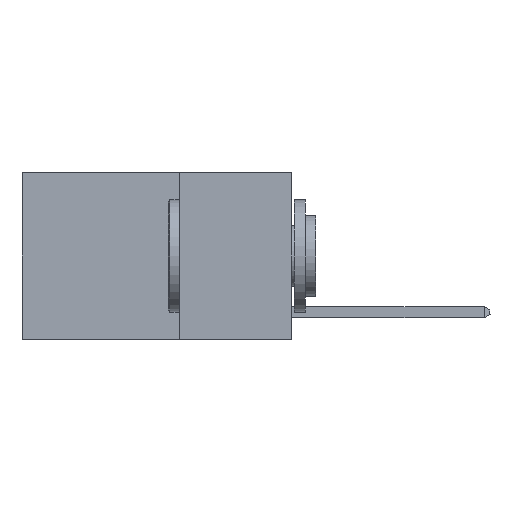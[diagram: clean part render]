
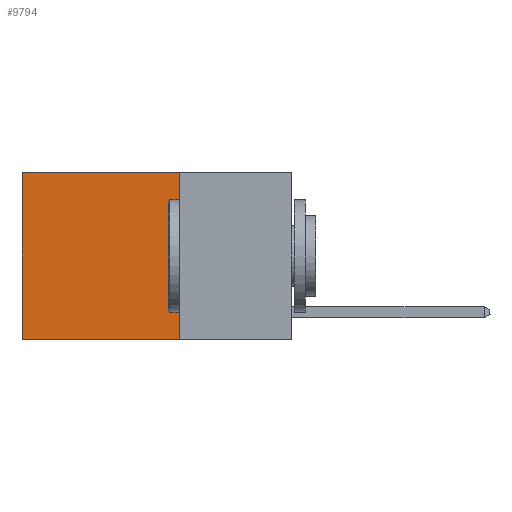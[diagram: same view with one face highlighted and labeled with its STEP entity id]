
A CAD part, left-side view. The second image highlights one B-rep face of the part: STEP entity #9794.
In plain terms, the highlighted planar face has unit normal (-1, 0, 0).
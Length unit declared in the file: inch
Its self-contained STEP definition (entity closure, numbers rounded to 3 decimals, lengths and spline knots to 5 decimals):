
#25 = ORIENTED_EDGE ( 'NONE', *, *, #17790, .T. ) ;
#672 = ORIENTED_EDGE ( 'NONE', *, *, #15250, .F. ) ;
#1706 = CARTESIAN_POINT ( 'NONE',  ( 0.2625, 0.25, 0. ) ) ;
#1743 = ORIENTED_EDGE ( 'NONE', *, *, #19014, .T. ) ;
#1976 = CARTESIAN_POINT ( 'NONE',  ( 0.2625, 0.6, 0. ) ) ;
#2113 = VERTEX_POINT ( 'NONE', #15610 ) ;
#3565 = CARTESIAN_POINT ( 'NONE',  ( 0.2625, 0.25, 0. ) ) ;
#3771 = VECTOR ( 'NONE', #5087, 39.37008 ) ;
#3890 = VERTEX_POINT ( 'NONE', #6800 ) ;
#5020 = CARTESIAN_POINT ( 'NONE',  ( 0.2625, 0.25, 0. ) ) ;
#5087 = DIRECTION ( 'NONE',  ( 0., 0., -1. ) ) ;
#5312 = DIRECTION ( 'NONE',  ( 0., 0., -1. ) ) ;
#5803 = VECTOR ( 'NONE', #11676, 39.37008 ) ;
#6051 = VERTEX_POINT ( 'NONE', #1976 ) ;
#6800 = CARTESIAN_POINT ( 'NONE',  ( 0.2625, 0.25, -0.37 ) ) ;
#7017 = VECTOR ( 'NONE', #13240, 39.37008 ) ;
#7390 = ORIENTED_EDGE ( 'NONE', *, *, #19089, .F. ) ;
#7857 = FACE_OUTER_BOUND ( 'NONE', #13438, .T. ) ;
#8867 = CARTESIAN_POINT ( 'NONE',  ( 0.2625, 0.6, -0.37 ) ) ;
#9794 = ADVANCED_FACE ( 'NONE', ( #7857 ), #11970, .F. ) ;
#10110 = CARTESIAN_POINT ( 'NONE',  ( 0.2625, 0.6, 0. ) ) ;
#11676 = DIRECTION ( 'NONE',  ( 0., 1., 0. ) ) ;
#11970 = PLANE ( 'NONE',  #16778 ) ;
#13240 = DIRECTION ( 'NONE',  ( 0., 1., 0. ) ) ;
#13438 = EDGE_LOOP ( 'NONE', ( #25, #672, #7390, #1743 ) ) ;
#14285 = VECTOR ( 'NONE', #15061, 39.37008 ) ;
#14671 = LINE ( 'NONE', #16667, #5803 ) ;
#15061 = DIRECTION ( 'NONE',  ( 0., 0., -1. ) ) ;
#15250 = EDGE_CURVE ( 'NONE', #3890, #21737, #14671, .T. ) ;
#15346 = DIRECTION ( 'NONE',  ( 1., 0., 0. ) ) ;
#15610 = CARTESIAN_POINT ( 'NONE',  ( 0.2625, 0.25, 0. ) ) ;
#16667 = CARTESIAN_POINT ( 'NONE',  ( 0.2625, 0.25, -0.37 ) ) ;
#16778 = AXIS2_PLACEMENT_3D ( 'NONE', #3565, #15346, #5312 ) ;
#17731 = LINE ( 'NONE', #10110, #3771 ) ;
#17790 = EDGE_CURVE ( 'NONE', #6051, #21737, #17731, .T. ) ;
#18772 = LINE ( 'NONE', #5020, #14285 ) ;
#19014 = EDGE_CURVE ( 'NONE', #2113, #6051, #20321, .T. ) ;
#19089 = EDGE_CURVE ( 'NONE', #2113, #3890, #18772, .T. ) ;
#20321 = LINE ( 'NONE', #1706, #7017 ) ;
#21737 = VERTEX_POINT ( 'NONE', #8867 ) ;
